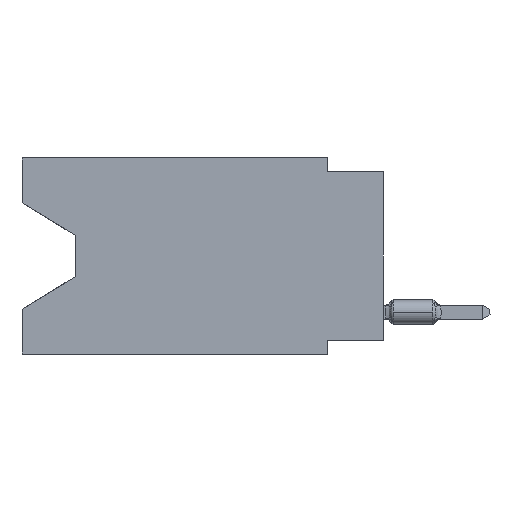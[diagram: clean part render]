
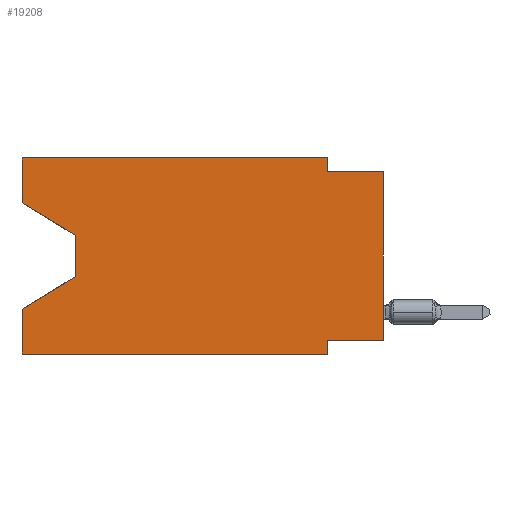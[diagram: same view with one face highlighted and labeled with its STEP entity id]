
A CAD part, left-side view. The second image highlights one B-rep face of the part: STEP entity #19208.
In plain terms, the highlighted planar face has unit normal (-1, 0, 0).
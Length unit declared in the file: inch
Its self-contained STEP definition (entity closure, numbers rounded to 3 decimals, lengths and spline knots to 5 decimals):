
#385 = DIRECTION ( 'NONE',  ( 0., -0.855, -0.519 ) ) ;
#615 = EDGE_CURVE ( 'NONE', #3658, #15193, #6332, .T. ) ;
#632 = EDGE_CURVE ( 'NONE', #18918, #1032, #4865, .T. ) ;
#1032 = VERTEX_POINT ( 'NONE', #6506 ) ;
#1320 = DIRECTION ( 'NONE',  ( 0., -1., 0. ) ) ;
#1783 = LINE ( 'NONE', #10623, #3611 ) ;
#1852 = CARTESIAN_POINT ( 'NONE',  ( 0., 0.1, -0.325 ) ) ;
#1980 = CARTESIAN_POINT ( 'NONE',  ( 0., 0., -0.325 ) ) ;
#2119 = EDGE_CURVE ( 'NONE', #4349, #18918, #13916, .T. ) ;
#2189 = VERTEX_POINT ( 'NONE', #1852 ) ;
#2455 = VECTOR ( 'NONE', #18517, 39.37008 ) ;
#2457 = DIRECTION ( 'NONE',  ( 0., 0., -1. ) ) ;
#2782 = LINE ( 'NONE', #16338, #9212 ) ;
#2868 = EDGE_CURVE ( 'NONE', #3658, #1032, #10735, .T. ) ;
#2995 = ORIENTED_EDGE ( 'NONE', *, *, #2868, .F. ) ;
#3113 = ORIENTED_EDGE ( 'NONE', *, *, #18334, .F. ) ;
#3611 = VECTOR ( 'NONE', #385, 39.37008 ) ;
#3658 = VERTEX_POINT ( 'NONE', #16867 ) ;
#3942 = DIRECTION ( 'NONE',  ( 0., -1., 0. ) ) ;
#4211 = DIRECTION ( 'NONE',  ( 0., 0., -1. ) ) ;
#4253 = ORIENTED_EDGE ( 'NONE', *, *, #12740, .F. ) ;
#4318 = DIRECTION ( 'NONE',  ( 0., 0., 1. ) ) ;
#4349 = VERTEX_POINT ( 'NONE', #13168 ) ;
#4474 = ORIENTED_EDGE ( 'NONE', *, *, #5154, .F. ) ;
#4829 = CARTESIAN_POINT ( 'NONE',  ( 0., 0.55, -0.212 ) ) ;
#4865 = LINE ( 'NONE', #10854, #16501 ) ;
#4994 = CARTESIAN_POINT ( 'NONE',  ( 0., 0.55, -0.138 ) ) ;
#5154 = EDGE_CURVE ( 'NONE', #17219, #10654, #5573, .T. ) ;
#5573 = LINE ( 'NONE', #7143, #9428 ) ;
#6099 = ORIENTED_EDGE ( 'NONE', *, *, #15264, .F. ) ;
#6103 = ORIENTED_EDGE ( 'NONE', *, *, #7505, .F. ) ;
#6135 = VECTOR ( 'NONE', #17810, 39.37008 ) ;
#6332 = LINE ( 'NONE', #12309, #8024 ) ;
#6476 = AXIS2_PLACEMENT_3D ( 'NONE', #17658, #10204, #2457 ) ;
#6506 = CARTESIAN_POINT ( 'NONE',  ( 0., 0.645, -0.26975 ) ) ;
#6762 = CARTESIAN_POINT ( 'NONE',  ( 0., 0.1, 0. ) ) ;
#6848 = VERTEX_POINT ( 'NONE', #6762 ) ;
#6964 = CARTESIAN_POINT ( 'NONE',  ( 0., 0.1, -0.35 ) ) ;
#7143 = CARTESIAN_POINT ( 'NONE',  ( 0., 0., -0.025 ) ) ;
#7378 = ORIENTED_EDGE ( 'NONE', *, *, #632, .T. ) ;
#7505 = EDGE_CURVE ( 'NONE', #6848, #17219, #8843, .T. ) ;
#7823 = EDGE_CURVE ( 'NONE', #17371, #10654, #15113, .T. ) ;
#7887 = DIRECTION ( 'NONE',  ( 0., 0., 1. ) ) ;
#8024 = VECTOR ( 'NONE', #18298, 39.37008 ) ;
#8843 = LINE ( 'NONE', #14841, #10420 ) ;
#9212 = VECTOR ( 'NONE', #10041, 39.37008 ) ;
#9380 = DIRECTION ( 'NONE',  ( 0., 0.855, -0.519 ) ) ;
#9381 = ORIENTED_EDGE ( 'NONE', *, *, #615, .T. ) ;
#9428 = VECTOR ( 'NONE', #1320, 39.37008 ) ;
#10004 = LINE ( 'NONE', #6964, #12093 ) ;
#10041 = DIRECTION ( 'NONE',  ( 0., 0., 1. ) ) ;
#10142 = CARTESIAN_POINT ( 'NONE',  ( 0., 0.1, -0.025 ) ) ;
#10204 = DIRECTION ( 'NONE',  ( 1., 0., 0. ) ) ;
#10420 = VECTOR ( 'NONE', #15339, 39.37008 ) ;
#10597 = ORIENTED_EDGE ( 'NONE', *, *, #18829, .T. ) ;
#10623 = CARTESIAN_POINT ( 'NONE',  ( 0., 0.645, -0.08025 ) ) ;
#10654 = VERTEX_POINT ( 'NONE', #11900 ) ;
#10735 = LINE ( 'NONE', #18100, #17335 ) ;
#10765 = VECTOR ( 'NONE', #4318, 39.37008 ) ;
#10854 = CARTESIAN_POINT ( 'NONE',  ( 0., 0.55, -0.212 ) ) ;
#11223 = ORIENTED_EDGE ( 'NONE', *, *, #2119, .T. ) ;
#11403 = CARTESIAN_POINT ( 'NONE',  ( 0., 0.645, 0. ) ) ;
#11664 = PLANE ( 'NONE',  #6476 ) ;
#11900 = CARTESIAN_POINT ( 'NONE',  ( 0., 0., -0.025 ) ) ;
#12016 = EDGE_LOOP ( 'NONE', ( #10597, #11223, #7378, #2995, #9381, #4253, #3113, #16961, #4474, #6103, #6099, #14383 ) ) ;
#12093 = VECTOR ( 'NONE', #4211, 39.37008 ) ;
#12309 = CARTESIAN_POINT ( 'NONE',  ( 0., 0.645, -0.35 ) ) ;
#12740 = EDGE_CURVE ( 'NONE', #2189, #15193, #10004, .T. ) ;
#12907 = VERTEX_POINT ( 'NONE', #16588 ) ;
#13168 = CARTESIAN_POINT ( 'NONE',  ( 0., 0.55, -0.138 ) ) ;
#13187 = LINE ( 'NONE', #16041, #6135 ) ;
#13653 = VERTEX_POINT ( 'NONE', #15954 ) ;
#13916 = LINE ( 'NONE', #4994, #2455 ) ;
#14383 = ORIENTED_EDGE ( 'NONE', *, *, #14793, .F. ) ;
#14793 = EDGE_CURVE ( 'NONE', #13653, #12907, #2782, .T. ) ;
#14841 = CARTESIAN_POINT ( 'NONE',  ( 0., 0.1, 0. ) ) ;
#15020 = CARTESIAN_POINT ( 'NONE',  ( 0., 0., 0. ) ) ;
#15113 = LINE ( 'NONE', #15020, #10765 ) ;
#15193 = VERTEX_POINT ( 'NONE', #15936 ) ;
#15264 = EDGE_CURVE ( 'NONE', #12907, #6848, #18855, .T. ) ;
#15339 = DIRECTION ( 'NONE',  ( 0., 0., -1. ) ) ;
#15764 = VECTOR ( 'NONE', #3942, 39.37008 ) ;
#15921 = FACE_OUTER_BOUND ( 'NONE', #12016, .T. ) ;
#15936 = CARTESIAN_POINT ( 'NONE',  ( 0., 0.1, -0.35 ) ) ;
#15954 = CARTESIAN_POINT ( 'NONE',  ( 0., 0.645, -0.08025 ) ) ;
#16041 = CARTESIAN_POINT ( 'NONE',  ( 0., 0., -0.325 ) ) ;
#16338 = CARTESIAN_POINT ( 'NONE',  ( 0., 0.645, 0. ) ) ;
#16501 = VECTOR ( 'NONE', #9380, 39.37008 ) ;
#16588 = CARTESIAN_POINT ( 'NONE',  ( 0., 0.645, 0. ) ) ;
#16867 = CARTESIAN_POINT ( 'NONE',  ( 0., 0.645, -0.35 ) ) ;
#16961 = ORIENTED_EDGE ( 'NONE', *, *, #7823, .T. ) ;
#17219 = VERTEX_POINT ( 'NONE', #10142 ) ;
#17335 = VECTOR ( 'NONE', #7887, 39.37008 ) ;
#17371 = VERTEX_POINT ( 'NONE', #1980 ) ;
#17658 = CARTESIAN_POINT ( 'NONE',  ( 0., 0.645, 0. ) ) ;
#17810 = DIRECTION ( 'NONE',  ( 0., 1., 0. ) ) ;
#18100 = CARTESIAN_POINT ( 'NONE',  ( 0., 0.645, 0. ) ) ;
#18298 = DIRECTION ( 'NONE',  ( 0., -1., 0. ) ) ;
#18334 = EDGE_CURVE ( 'NONE', #17371, #2189, #13187, .T. ) ;
#18517 = DIRECTION ( 'NONE',  ( 0., 0., -1. ) ) ;
#18829 = EDGE_CURVE ( 'NONE', #13653, #4349, #1783, .T. ) ;
#18855 = LINE ( 'NONE', #11403, #15764 ) ;
#18918 = VERTEX_POINT ( 'NONE', #4829 ) ;
#19208 = ADVANCED_FACE ( 'NONE', ( #15921 ), #11664, .F. ) ;
